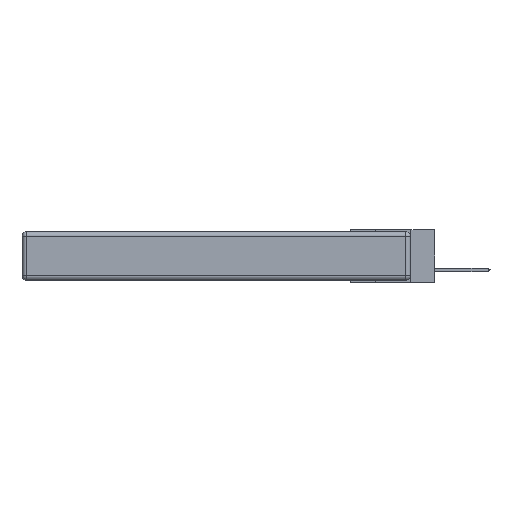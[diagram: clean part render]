
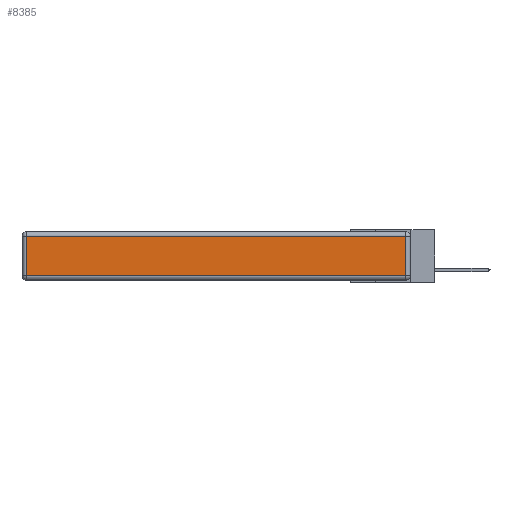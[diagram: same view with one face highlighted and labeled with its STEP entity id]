
A CAD part, left-side view. The second image highlights one B-rep face of the part: STEP entity #8385.
In plain terms, the highlighted planar face has unit normal (-1, 0, 0).
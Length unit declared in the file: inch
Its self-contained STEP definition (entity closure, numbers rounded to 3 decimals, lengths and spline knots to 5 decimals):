
#22 = AXIS2_PLACEMENT_3D ( 'NONE', #4286, #8211, #9195 ) ;
#320 = DIRECTION ( 'NONE',  ( 0., -1., 0. ) ) ;
#2763 = VERTEX_POINT ( 'NONE', #8744 ) ;
#3265 = PLANE ( 'NONE',  #22 ) ;
#3593 = FACE_OUTER_BOUND ( 'NONE', #10168, .T. ) ;
#3615 = VECTOR ( 'NONE', #9624, 39.37008 ) ;
#4286 = CARTESIAN_POINT ( 'NONE',  ( 0., 0., -0.343 ) ) ;
#4309 = CARTESIAN_POINT ( 'NONE',  ( 0., 0., -0.313 ) ) ;
#4769 = VECTOR ( 'NONE', #8529, 39.37008 ) ;
#5028 = EDGE_CURVE ( 'NONE', #5754, #2763, #6665, .T. ) ;
#5030 = CARTESIAN_POINT ( 'NONE',  ( 0., 2.75, -0.03 ) ) ;
#5396 = CARTESIAN_POINT ( 'NONE',  ( 0., 2.72, -0.03 ) ) ;
#5754 = VERTEX_POINT ( 'NONE', #5396 ) ;
#6665 = LINE ( 'NONE', #11640, #3615 ) ;
#7560 = EDGE_CURVE ( 'NONE', #2763, #9139, #8361, .T. ) ;
#7830 = CARTESIAN_POINT ( 'NONE',  ( 0., 0.03, -0.313 ) ) ;
#7874 = VECTOR ( 'NONE', #11811, 39.37008 ) ;
#8019 = LINE ( 'NONE', #5030, #7874 ) ;
#8211 = DIRECTION ( 'NONE',  ( -1., 0., 0. ) ) ;
#8232 = EDGE_CURVE ( 'NONE', #8411, #5754, #8019, .T. ) ;
#8361 = LINE ( 'NONE', #4309, #8677 ) ;
#8385 = ADVANCED_FACE ( 'NONE', ( #3593 ), #3265, .T. ) ;
#8411 = VERTEX_POINT ( 'NONE', #9609 ) ;
#8529 = DIRECTION ( 'NONE',  ( 0., 0., 1. ) ) ;
#8677 = VECTOR ( 'NONE', #320, 39.37008 ) ;
#8744 = CARTESIAN_POINT ( 'NONE',  ( 0., 2.72, -0.313 ) ) ;
#9139 = VERTEX_POINT ( 'NONE', #7830 ) ;
#9195 = DIRECTION ( 'NONE',  ( 0., 0., 1. ) ) ;
#9545 = ORIENTED_EDGE ( 'NONE', *, *, #7560, .T. ) ;
#9609 = CARTESIAN_POINT ( 'NONE',  ( 0., 0.03, -0.03 ) ) ;
#9624 = DIRECTION ( 'NONE',  ( 0., 0., -1. ) ) ;
#9795 = ORIENTED_EDGE ( 'NONE', *, *, #10175, .T. ) ;
#9850 = LINE ( 'NONE', #11309, #4769 ) ;
#10168 = EDGE_LOOP ( 'NONE', ( #9545, #9795, #10438, #10871 ) ) ;
#10175 = EDGE_CURVE ( 'NONE', #9139, #8411, #9850, .T. ) ;
#10438 = ORIENTED_EDGE ( 'NONE', *, *, #8232, .T. ) ;
#10871 = ORIENTED_EDGE ( 'NONE', *, *, #5028, .T. ) ;
#11309 = CARTESIAN_POINT ( 'NONE',  ( 0., 0.03, -0.343 ) ) ;
#11640 = CARTESIAN_POINT ( 'NONE',  ( 0., 2.72, -0.343 ) ) ;
#11811 = DIRECTION ( 'NONE',  ( 0., 1., 0. ) ) ;
